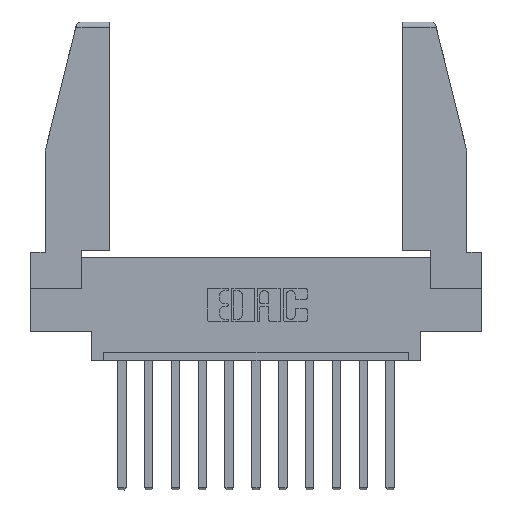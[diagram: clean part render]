
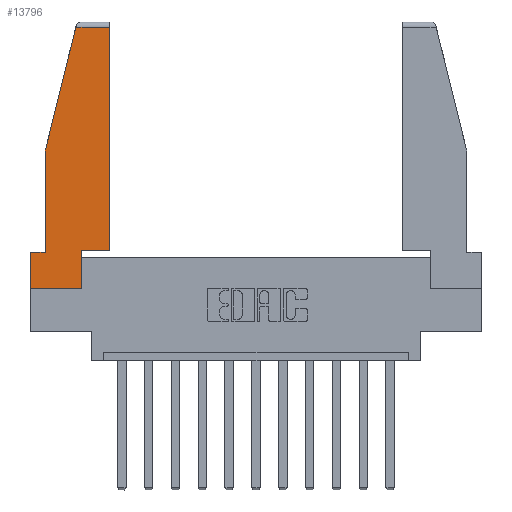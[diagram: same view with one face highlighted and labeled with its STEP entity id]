
A CAD part, top view. The second image highlights one B-rep face of the part: STEP entity #13796.
In plain terms, the highlighted planar face has unit normal (0, 0, 1).
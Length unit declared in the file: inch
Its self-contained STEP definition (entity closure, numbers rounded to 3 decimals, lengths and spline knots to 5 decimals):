
#68 = CARTESIAN_POINT ( 'NONE',  ( 0., 0., 0. ) ) ;
#174 = CARTESIAN_POINT ( 'NONE',  ( 0.086, 0.8, 0. ) ) ;
#199 = CARTESIAN_POINT ( 'NONE',  ( 0.461, 0.223, 0. ) ) ;
#311 = VECTOR ( 'NONE', #11732, 39.37008 ) ;
#430 = DIRECTION ( 'NONE',  ( 0., 0., 1. ) ) ;
#724 = ORIENTED_EDGE ( 'NONE', *, *, #5903, .T. ) ;
#769 = ORIENTED_EDGE ( 'NONE', *, *, #4850, .T. ) ;
#934 = VERTEX_POINT ( 'NONE', #199 ) ;
#1056 = DIRECTION ( 'NONE',  ( 1., 0., 0. ) ) ;
#1097 = AXIS2_PLACEMENT_3D ( 'NONE', #5995, #430, #8630 ) ;
#1128 = VECTOR ( 'NONE', #1056, 39.37008 ) ;
#1405 = CARTESIAN_POINT ( 'NONE',  ( 0.086, 0.21, 0. ) ) ;
#1466 = CARTESIAN_POINT ( 'NONE',  ( 0.297, 0.223, 0. ) ) ;
#1485 = LINE ( 'NONE', #68, #1128 ) ;
#1834 = CARTESIAN_POINT ( 'NONE',  ( 0.271, 1.55, 0. ) ) ;
#1862 = VECTOR ( 'NONE', #4183, 39.37008 ) ;
#1907 = VERTEX_POINT ( 'NONE', #4341 ) ;
#2062 = DIRECTION ( 'NONE',  ( 1., 0., 0. ) ) ;
#2484 = ORIENTED_EDGE ( 'NONE', *, *, #8409, .T. ) ;
#2679 = EDGE_CURVE ( 'NONE', #7608, #5171, #1485, .T. ) ;
#3496 = VECTOR ( 'NONE', #5711, 39.37008 ) ;
#3958 = LINE ( 'NONE', #6462, #1862 ) ;
#4109 = LINE ( 'NONE', #8981, #6936 ) ;
#4183 = DIRECTION ( 'NONE',  ( 0., -1., 0. ) ) ;
#4306 = CARTESIAN_POINT ( 'NONE',  ( 0.461, 1.52, 0. ) ) ;
#4341 = CARTESIAN_POINT ( 'NONE',  ( 0.2636, 1.52, 0. ) ) ;
#4380 = LINE ( 'NONE', #13580, #3496 ) ;
#4826 = ORIENTED_EDGE ( 'NONE', *, *, #4993, .T. ) ;
#4850 = EDGE_CURVE ( 'NONE', #934, #12152, #5107, .T. ) ;
#4993 = EDGE_CURVE ( 'NONE', #7606, #6501, #4380, .T. ) ;
#5107 = LINE ( 'NONE', #7839, #7586 ) ;
#5171 = VERTEX_POINT ( 'NONE', #5205 ) ;
#5205 = CARTESIAN_POINT ( 'NONE',  ( 0.297, 0., 0. ) ) ;
#5711 = DIRECTION ( 'NONE',  ( -1., 0., 0. ) ) ;
#5732 = VERTEX_POINT ( 'NONE', #12268 ) ;
#5903 = EDGE_CURVE ( 'NONE', #5732, #7606, #11220, .T. ) ;
#5995 = CARTESIAN_POINT ( 'NONE',  ( 0., 0., 0. ) ) ;
#6126 = LINE ( 'NONE', #1834, #14093 ) ;
#6329 = ORIENTED_EDGE ( 'NONE', *, *, #2679, .T. ) ;
#6462 = CARTESIAN_POINT ( 'NONE',  ( 0., 0.21, 0. ) ) ;
#6501 = VERTEX_POINT ( 'NONE', #14346 ) ;
#6697 = EDGE_CURVE ( 'NONE', #1907, #5732, #6126, .T. ) ;
#6936 = VECTOR ( 'NONE', #2062, 39.37008 ) ;
#7259 = CARTESIAN_POINT ( 'NONE',  ( 0.297, 0., 0. ) ) ;
#7326 = ORIENTED_EDGE ( 'NONE', *, *, #10423, .T. ) ;
#7586 = VECTOR ( 'NONE', #8965, 39.37008 ) ;
#7606 = VERTEX_POINT ( 'NONE', #1405 ) ;
#7608 = VERTEX_POINT ( 'NONE', #14075 ) ;
#7630 = ORIENTED_EDGE ( 'NONE', *, *, #9600, .T. ) ;
#7839 = CARTESIAN_POINT ( 'NONE',  ( 0.461, 0.223, 0. ) ) ;
#8017 = DIRECTION ( 'NONE',  ( 0., -1., 0. ) ) ;
#8368 = DIRECTION ( 'NONE',  ( -0.239, -0.971, 0. ) ) ;
#8409 = EDGE_CURVE ( 'NONE', #5171, #11137, #10130, .T. ) ;
#8602 = VECTOR ( 'NONE', #12623, 39.37008 ) ;
#8630 = DIRECTION ( 'NONE',  ( 1., 0., 0. ) ) ;
#8921 = EDGE_LOOP ( 'NONE', ( #769, #13411, #12349, #724, #4826, #7630, #6329, #2484, #7326 ) ) ;
#8965 = DIRECTION ( 'NONE',  ( 0., 1., 0. ) ) ;
#8981 = CARTESIAN_POINT ( 'NONE',  ( 0.297, 0.223, 0. ) ) ;
#9600 = EDGE_CURVE ( 'NONE', #6501, #7608, #3958, .T. ) ;
#10130 = LINE ( 'NONE', #7259, #311 ) ;
#10423 = EDGE_CURVE ( 'NONE', #11137, #934, #4109, .T. ) ;
#11137 = VERTEX_POINT ( 'NONE', #1466 ) ;
#11220 = LINE ( 'NONE', #174, #11965 ) ;
#11732 = DIRECTION ( 'NONE',  ( 0., 1., 0. ) ) ;
#11951 = FACE_OUTER_BOUND ( 'NONE', #8921, .T. ) ;
#11965 = VECTOR ( 'NONE', #8017, 39.37008 ) ;
#12152 = VERTEX_POINT ( 'NONE', #4306 ) ;
#12268 = CARTESIAN_POINT ( 'NONE',  ( 0.086, 0.8, 0. ) ) ;
#12349 = ORIENTED_EDGE ( 'NONE', *, *, #6697, .T. ) ;
#12623 = DIRECTION ( 'NONE',  ( -1., 0., 0. ) ) ;
#12766 = PLANE ( 'NONE',  #1097 ) ;
#12948 = EDGE_CURVE ( 'NONE', #12152, #1907, #13734, .T. ) ;
#13411 = ORIENTED_EDGE ( 'NONE', *, *, #12948, .T. ) ;
#13580 = CARTESIAN_POINT ( 'NONE',  ( 0., 0.21, 0. ) ) ;
#13734 = LINE ( 'NONE', #13812, #8602 ) ;
#13796 = ADVANCED_FACE ( 'NONE', ( #11951 ), #12766, .T. ) ;
#13812 = CARTESIAN_POINT ( 'NONE',  ( 0., 1.52, 0. ) ) ;
#14075 = CARTESIAN_POINT ( 'NONE',  ( 0., 0., 0. ) ) ;
#14093 = VECTOR ( 'NONE', #8368, 39.37008 ) ;
#14346 = CARTESIAN_POINT ( 'NONE',  ( 0., 0.21, 0. ) ) ;
